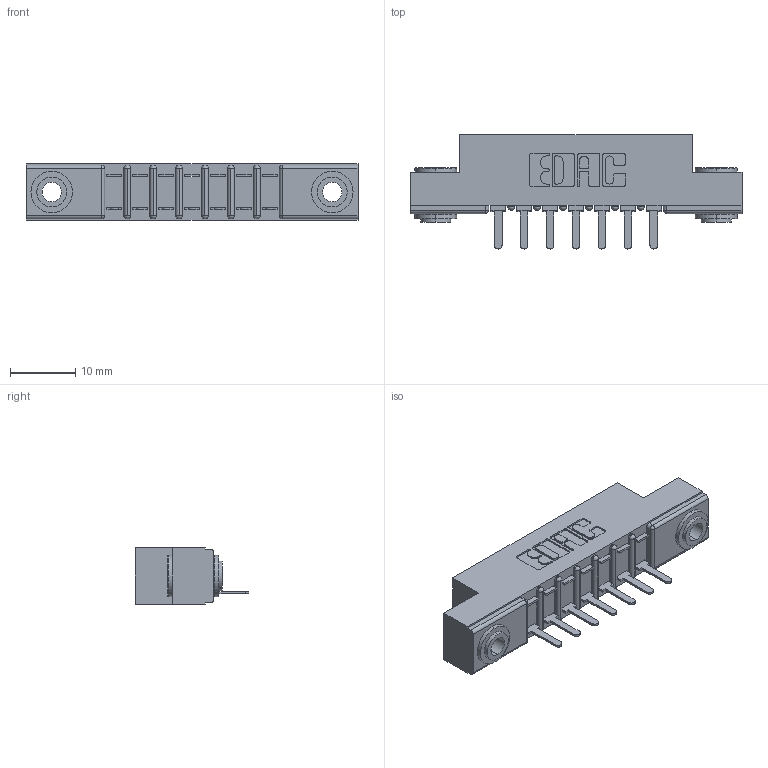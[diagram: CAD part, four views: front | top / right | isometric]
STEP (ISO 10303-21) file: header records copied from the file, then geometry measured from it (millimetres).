
FILE_DESCRIPTION (( 'STEP AP203' ), '1' );
FILE_NAME ('307-007-421-103.STEP', '2020-09-25T02:15:55', ( '' ), ( '' ), 'SwSTEP 2.0', 'SolidWorks 2020', '' );
FILE_SCHEMA (( 'CONFIG_CONTROL_DESIGN' ));
Length unit declared in the file: inch
Products named in the file (4): 307-007-421-103; 345-250-002_345-250-002-102; 307-290-002_521; 307 Part_.156 Dia Mounting Holes
Assembly tree (10 placements, depth 2):
  307-007-421-103
    307 Part_.156 Dia Mounting Holes
    307-290-002_521  x7
    345-250-002_345-250-002-102  x2
Bounding box: 50.75 x 17.42 x 8.71 mm (x, y, z)
Volume: 3344.2 mm3; surface area: 5496.7 mm2
Topology: 10 solids, 10 shells, 696 faces, 2059 edges, 1346 vertices
Faces by surface type: plane 409, cylinder 263, sphere 16, cone 8
Entity records: 12099 total; most frequent: CARTESIAN_POINT 2013, ORIENTED_EDGE 1994, DIRECTION 1987, EDGE_CURVE 997, LINE 739, VECTOR 739, VERTEX_POINT 650, AXIS2_PLACEMENT_3D 624
